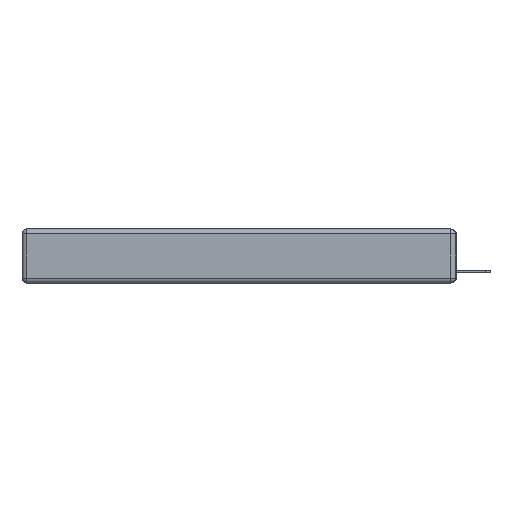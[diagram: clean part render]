
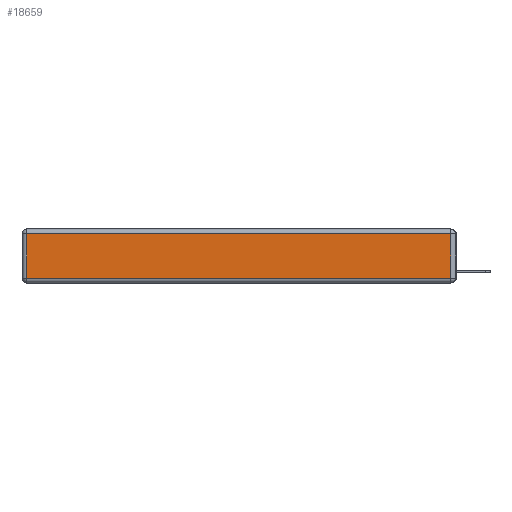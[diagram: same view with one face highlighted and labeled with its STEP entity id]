
A CAD part, left-side view. The second image highlights one B-rep face of the part: STEP entity #18659.
In plain terms, the highlighted planar face has unit normal (-1, 0, 0).
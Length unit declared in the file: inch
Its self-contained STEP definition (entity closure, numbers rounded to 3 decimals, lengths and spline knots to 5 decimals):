
#289 = VECTOR ( 'NONE', #4645, 39.37008 ) ;
#1834 = EDGE_CURVE ( 'NONE', #26968, #17206, #14799, .T. ) ;
#2360 = LINE ( 'NONE', #26263, #25847 ) ;
#3466 = CARTESIAN_POINT ( 'NONE',  ( 0., 0.03, -0.313 ) ) ;
#4546 = CARTESIAN_POINT ( 'NONE',  ( 0., 0., -0.313 ) ) ;
#4645 = DIRECTION ( 'NONE',  ( 0., -1., 0. ) ) ;
#5941 = VERTEX_POINT ( 'NONE', #14069 ) ;
#7928 = VECTOR ( 'NONE', #12349, 39.37008 ) ;
#8268 = CARTESIAN_POINT ( 'NONE',  ( 0., 0., -0.343 ) ) ;
#8610 = DIRECTION ( 'NONE',  ( 0., 0., 1. ) ) ;
#11024 = EDGE_CURVE ( 'NONE', #5941, #12235, #27187, .T. ) ;
#12235 = VERTEX_POINT ( 'NONE', #27773 ) ;
#12349 = DIRECTION ( 'NONE',  ( 0., 0., -1. ) ) ;
#12718 = DIRECTION ( 'NONE',  ( 0., 0., 1. ) ) ;
#13319 = CARTESIAN_POINT ( 'NONE',  ( 0., 2.72, -0.313 ) ) ;
#13851 = EDGE_LOOP ( 'NONE', ( #25718, #25113, #13964, #25712 ) ) ;
#13964 = ORIENTED_EDGE ( 'NONE', *, *, #11024, .T. ) ;
#14069 = CARTESIAN_POINT ( 'NONE',  ( 0., 0.03, -0.03 ) ) ;
#14799 = LINE ( 'NONE', #4546, #289 ) ;
#15106 = PLANE ( 'NONE',  #17525 ) ;
#17206 = VERTEX_POINT ( 'NONE', #3466 ) ;
#17525 = AXIS2_PLACEMENT_3D ( 'NONE', #8268, #19217, #12718 ) ;
#18659 = ADVANCED_FACE ( 'NONE', ( #22437 ), #15106, .T. ) ;
#19217 = DIRECTION ( 'NONE',  ( -1., 0., 0. ) ) ;
#22075 = LINE ( 'NONE', #28041, #7928 ) ;
#22437 = FACE_OUTER_BOUND ( 'NONE', #13851, .T. ) ;
#22638 = CARTESIAN_POINT ( 'NONE',  ( 0., 2.75, -0.03 ) ) ;
#24660 = DIRECTION ( 'NONE',  ( 0., 1., 0. ) ) ;
#25113 = ORIENTED_EDGE ( 'NONE', *, *, #28231, .T. ) ;
#25712 = ORIENTED_EDGE ( 'NONE', *, *, #27470, .T. ) ;
#25718 = ORIENTED_EDGE ( 'NONE', *, *, #1834, .T. ) ;
#25847 = VECTOR ( 'NONE', #8610, 39.37008 ) ;
#26176 = VECTOR ( 'NONE', #24660, 39.37008 ) ;
#26263 = CARTESIAN_POINT ( 'NONE',  ( 0., 0.03, -0.343 ) ) ;
#26968 = VERTEX_POINT ( 'NONE', #13319 ) ;
#27187 = LINE ( 'NONE', #22638, #26176 ) ;
#27470 = EDGE_CURVE ( 'NONE', #12235, #26968, #22075, .T. ) ;
#27773 = CARTESIAN_POINT ( 'NONE',  ( 0., 2.72, -0.03 ) ) ;
#28041 = CARTESIAN_POINT ( 'NONE',  ( 0., 2.72, -0.343 ) ) ;
#28231 = EDGE_CURVE ( 'NONE', #17206, #5941, #2360, .T. ) ;
